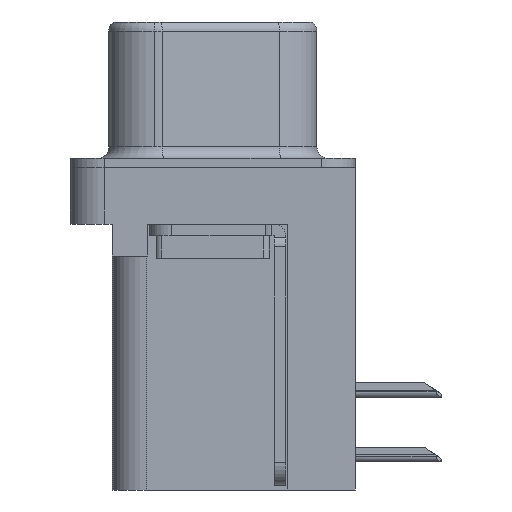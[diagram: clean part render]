
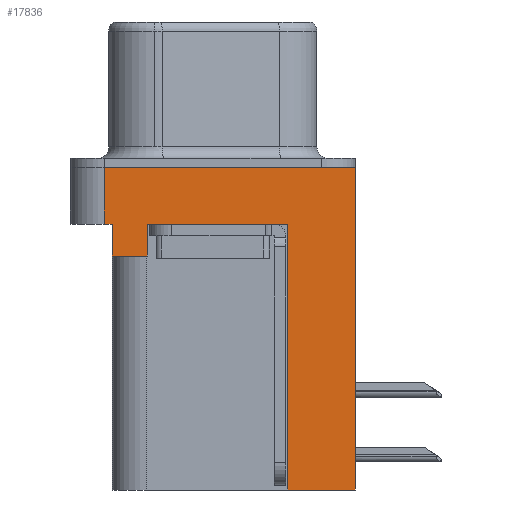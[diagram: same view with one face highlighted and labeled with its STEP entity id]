
A CAD part, left-side view. The second image highlights one B-rep face of the part: STEP entity #17836.
In plain terms, the highlighted planar face has unit normal (-1, 0, 0).
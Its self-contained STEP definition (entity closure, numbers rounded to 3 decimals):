
#269 = ORIENTED_EDGE ( 'NONE', *, *, #4925, .T. ) ;
#297 = CARTESIAN_POINT ( 'NONE',  ( -3., 4.425, -3.9 ) ) ;
#426 = ORIENTED_EDGE ( 'NONE', *, *, #16405, .F. ) ;
#537 = ORIENTED_EDGE ( 'NONE', *, *, #15410, .F. ) ;
#567 = AXIS2_PLACEMENT_3D ( 'NONE', #1728, #6001, #2510 ) ;
#644 = ORIENTED_EDGE ( 'NONE', *, *, #7840, .F. ) ;
#698 = VERTEX_POINT ( 'NONE', #16123 ) ;
#1030 = CARTESIAN_POINT ( 'NONE',  ( -3., 4.775, -2.5 ) ) ;
#1187 = CARTESIAN_POINT ( 'NONE',  ( -3., -3.295, -14.2 ) ) ;
#1625 = PLANE ( 'NONE',  #567 ) ;
#1728 = CARTESIAN_POINT ( 'NONE',  ( -3., -6.275, -2.5 ) ) ;
#2109 = EDGE_CURVE ( 'NONE', #4440, #14886, #9690, .T. ) ;
#2510 = DIRECTION ( 'NONE',  ( 0., 0., 1. ) ) ;
#2584 = DIRECTION ( 'NONE',  ( 0., -1., 0. ) ) ;
#2662 = CARTESIAN_POINT ( 'NONE',  ( -3., 2.895, -3.9 ) ) ;
#2689 = DIRECTION ( 'NONE',  ( 0., 1., 0. ) ) ;
#2930 = EDGE_CURVE ( 'NONE', #15354, #14638, #16475, .T. ) ;
#3322 = FACE_OUTER_BOUND ( 'NONE', #3543, .T. ) ;
#3419 = EDGE_CURVE ( 'NONE', #15354, #698, #20271, .T. ) ;
#3543 = EDGE_LOOP ( 'NONE', ( #16842, #21327, #11172, #644, #537, #22270, #269, #5117, #426, #18166 ) ) ;
#3594 = CARTESIAN_POINT ( 'NONE',  ( -3., -6.275, -2.5 ) ) ;
#4440 = VERTEX_POINT ( 'NONE', #11893 ) ;
#4680 = EDGE_CURVE ( 'NONE', #14638, #14886, #12751, .T. ) ;
#4711 = VECTOR ( 'NONE', #2584, 1000. ) ;
#4925 = EDGE_CURVE ( 'NONE', #6988, #8637, #13639, .T. ) ;
#5086 = LINE ( 'NONE', #6994, #20854 ) ;
#5117 = ORIENTED_EDGE ( 'NONE', *, *, #19361, .F. ) ;
#5484 = CARTESIAN_POINT ( 'NONE',  ( -3., -3.295, -2.5 ) ) ;
#5614 = CARTESIAN_POINT ( 'NONE',  ( -3., -6.275, 0. ) ) ;
#5718 = VECTOR ( 'NONE', #21744, 1000. ) ;
#6001 = DIRECTION ( 'NONE',  ( -1., 0., 0. ) ) ;
#6783 = DIRECTION ( 'NONE',  ( 0., 0., 1. ) ) ;
#6962 = DIRECTION ( 'NONE',  ( 0., -1., 0. ) ) ;
#6988 = VERTEX_POINT ( 'NONE', #20611 ) ;
#6994 = CARTESIAN_POINT ( 'NONE',  ( -3., 4.425, -3.9 ) ) ;
#7079 = CARTESIAN_POINT ( 'NONE',  ( -3., 4.775, 0. ) ) ;
#7166 = DIRECTION ( 'NONE',  ( 0., 1., 0. ) ) ;
#7840 = EDGE_CURVE ( 'NONE', #9220, #698, #5086, .T. ) ;
#7968 = CARTESIAN_POINT ( 'NONE',  ( -3., -3.295, -14.2 ) ) ;
#8456 = VECTOR ( 'NONE', #7166, 1000. ) ;
#8637 = VERTEX_POINT ( 'NONE', #5484 ) ;
#9220 = VERTEX_POINT ( 'NONE', #21758 ) ;
#9690 = LINE ( 'NONE', #14876, #5718 ) ;
#9917 = DIRECTION ( 'NONE',  ( 0., -1., 0. ) ) ;
#10192 = LINE ( 'NONE', #17064, #12350 ) ;
#11172 = ORIENTED_EDGE ( 'NONE', *, *, #3419, .T. ) ;
#11893 = CARTESIAN_POINT ( 'NONE',  ( -3., -6.275, -14.2 ) ) ;
#12350 = VECTOR ( 'NONE', #6783, 1000. ) ;
#12751 = LINE ( 'NONE', #16229, #4711 ) ;
#12913 = DIRECTION ( 'NONE',  ( 0., 0., 1. ) ) ;
#12954 = CARTESIAN_POINT ( 'NONE',  ( -3., -6.275, -2.5 ) ) ;
#13008 = EDGE_CURVE ( 'NONE', #19335, #6988, #10192, .T. ) ;
#13471 = VECTOR ( 'NONE', #9917, 1000. ) ;
#13639 = LINE ( 'NONE', #3594, #14169 ) ;
#13893 = DIRECTION ( 'NONE',  ( 0., 0., 1. ) ) ;
#14028 = VERTEX_POINT ( 'NONE', #16191 ) ;
#14169 = VECTOR ( 'NONE', #6962, 1000. ) ;
#14633 = VECTOR ( 'NONE', #2689, 1000. ) ;
#14638 = VERTEX_POINT ( 'NONE', #7079 ) ;
#14876 = CARTESIAN_POINT ( 'NONE',  ( -3., -6.275, -2.5 ) ) ;
#14886 = VERTEX_POINT ( 'NONE', #5614 ) ;
#15354 = VERTEX_POINT ( 'NONE', #17766 ) ;
#15410 = EDGE_CURVE ( 'NONE', #19335, #9220, #15752, .T. ) ;
#15752 = LINE ( 'NONE', #297, #8456 ) ;
#16123 = CARTESIAN_POINT ( 'NONE',  ( -3., 4.425, -2.5 ) ) ;
#16187 = LINE ( 'NONE', #1187, #16858 ) ;
#16191 = CARTESIAN_POINT ( 'NONE',  ( -3., -3.295, -14.2 ) ) ;
#16229 = CARTESIAN_POINT ( 'NONE',  ( -3., -6.275, 0. ) ) ;
#16405 = EDGE_CURVE ( 'NONE', #4440, #14028, #21727, .T. ) ;
#16475 = LINE ( 'NONE', #1030, #17270 ) ;
#16699 = DIRECTION ( 'NONE',  ( 0., 0., 1. ) ) ;
#16842 = ORIENTED_EDGE ( 'NONE', *, *, #4680, .F. ) ;
#16858 = VECTOR ( 'NONE', #12913, 1000. ) ;
#17064 = CARTESIAN_POINT ( 'NONE',  ( -3., 2.895, -3.9 ) ) ;
#17270 = VECTOR ( 'NONE', #16699, 1000. ) ;
#17766 = CARTESIAN_POINT ( 'NONE',  ( -3., 4.775, -2.5 ) ) ;
#17836 = ADVANCED_FACE ( 'NONE', ( #3322 ), #1625, .T. ) ;
#18166 = ORIENTED_EDGE ( 'NONE', *, *, #2109, .T. ) ;
#19335 = VERTEX_POINT ( 'NONE', #2662 ) ;
#19361 = EDGE_CURVE ( 'NONE', #14028, #8637, #16187, .T. ) ;
#20271 = LINE ( 'NONE', #12954, #13471 ) ;
#20611 = CARTESIAN_POINT ( 'NONE',  ( -3., 2.895, -2.5 ) ) ;
#20854 = VECTOR ( 'NONE', #13893, 1000. ) ;
#21327 = ORIENTED_EDGE ( 'NONE', *, *, #2930, .F. ) ;
#21727 = LINE ( 'NONE', #7968, #14633 ) ;
#21744 = DIRECTION ( 'NONE',  ( 0., 0., 1. ) ) ;
#21758 = CARTESIAN_POINT ( 'NONE',  ( -3., 4.425, -3.9 ) ) ;
#22270 = ORIENTED_EDGE ( 'NONE', *, *, #13008, .T. ) ;
